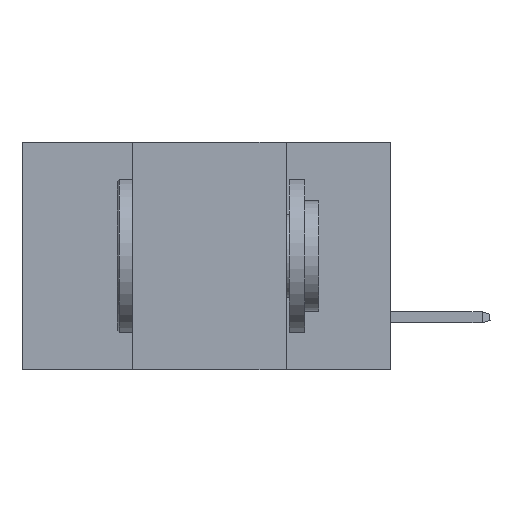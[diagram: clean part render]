
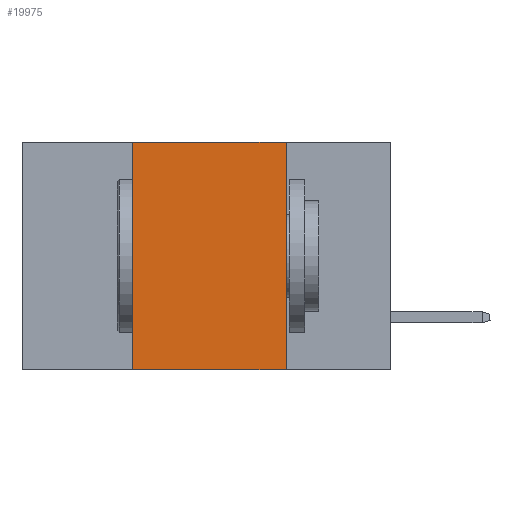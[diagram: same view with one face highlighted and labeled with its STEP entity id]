
A CAD part, left-side view. The second image highlights one B-rep face of the part: STEP entity #19975.
In plain terms, the highlighted planar face has unit normal (-1, 0, 0).
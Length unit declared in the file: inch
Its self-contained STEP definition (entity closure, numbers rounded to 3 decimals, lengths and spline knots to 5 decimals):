
#431 = ORIENTED_EDGE ( 'NONE', *, *, #21166, .F. ) ;
#1385 = CARTESIAN_POINT ( 'NONE',  ( 0., 0.17, 0. ) ) ;
#1468 = CARTESIAN_POINT ( 'NONE',  ( 0., 0.6, 0. ) ) ;
#1476 = PLANE ( 'NONE',  #3971 ) ;
#1669 = LINE ( 'NONE', #1385, #5579 ) ;
#2666 = CARTESIAN_POINT ( 'NONE',  ( 0., 0.17, -0.37 ) ) ;
#2806 = FACE_OUTER_BOUND ( 'NONE', #7760, .T. ) ;
#3417 = CARTESIAN_POINT ( 'NONE',  ( 0., 0.42, 0. ) ) ;
#3840 = DIRECTION ( 'NONE',  ( 1., 0., 0. ) ) ;
#3846 = ORIENTED_EDGE ( 'NONE', *, *, #4137, .F. ) ;
#3971 = AXIS2_PLACEMENT_3D ( 'NONE', #19915, #3840, #10892 ) ;
#4137 = EDGE_CURVE ( 'NONE', #23259, #6418, #14505, .T. ) ;
#4142 = VERTEX_POINT ( 'NONE', #2666 ) ;
#4447 = CARTESIAN_POINT ( 'NONE',  ( 0., 0.42, -0.37 ) ) ;
#5579 = VECTOR ( 'NONE', #26492, 39.37008 ) ;
#5885 = VECTOR ( 'NONE', #19720, 39.37008 ) ;
#6418 = VERTEX_POINT ( 'NONE', #3417 ) ;
#6508 = EDGE_CURVE ( 'NONE', #23259, #4142, #27517, .T. ) ;
#7760 = EDGE_LOOP ( 'NONE', ( #431, #11234, #3846, #27947 ) ) ;
#8538 = VECTOR ( 'NONE', #16226, 39.37008 ) ;
#8841 = EDGE_CURVE ( 'NONE', #6418, #24424, #27815, .T. ) ;
#10892 = DIRECTION ( 'NONE',  ( 0., 0., -1. ) ) ;
#11234 = ORIENTED_EDGE ( 'NONE', *, *, #8841, .F. ) ;
#11607 = CARTESIAN_POINT ( 'NONE',  ( 0., 0.17, 0. ) ) ;
#12310 = CARTESIAN_POINT ( 'NONE',  ( 0., 0.6, -0.37 ) ) ;
#14505 = LINE ( 'NONE', #18623, #8538 ) ;
#15111 = DIRECTION ( 'NONE',  ( 0., -1., 0. ) ) ;
#16226 = DIRECTION ( 'NONE',  ( 0., 0., 1. ) ) ;
#18623 = CARTESIAN_POINT ( 'NONE',  ( 0., 0.42, 0. ) ) ;
#19720 = DIRECTION ( 'NONE',  ( 0., -1., 0. ) ) ;
#19915 = CARTESIAN_POINT ( 'NONE',  ( 0., 0.6, 0. ) ) ;
#19975 = ADVANCED_FACE ( 'NONE', ( #2806 ), #1476, .F. ) ;
#21166 = EDGE_CURVE ( 'NONE', #24424, #4142, #1669, .T. ) ;
#21804 = VECTOR ( 'NONE', #15111, 39.37008 ) ;
#23259 = VERTEX_POINT ( 'NONE', #4447 ) ;
#24424 = VERTEX_POINT ( 'NONE', #11607 ) ;
#26492 = DIRECTION ( 'NONE',  ( 0., 0., -1. ) ) ;
#27517 = LINE ( 'NONE', #12310, #5885 ) ;
#27815 = LINE ( 'NONE', #1468, #21804 ) ;
#27947 = ORIENTED_EDGE ( 'NONE', *, *, #6508, .T. ) ;
